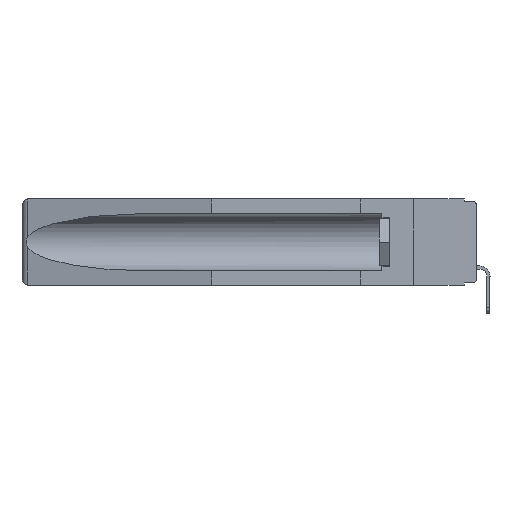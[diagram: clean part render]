
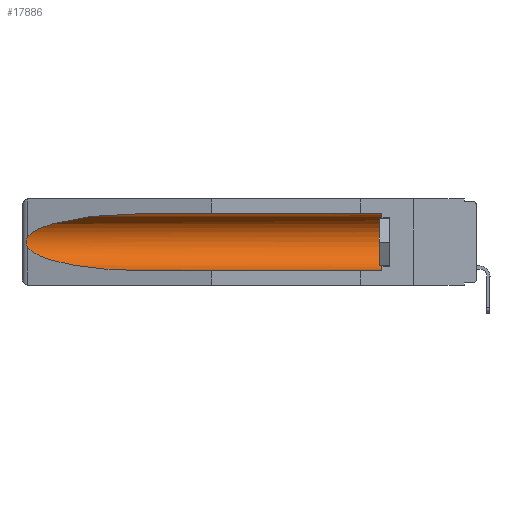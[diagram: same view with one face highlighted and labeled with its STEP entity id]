
A CAD part, left-side view. The second image highlights one B-rep face of the part: STEP entity #17886.
In plain terms, the highlighted cylindrical face has radius 2.857 mm (diameter 5.715 mm), a partial arc.
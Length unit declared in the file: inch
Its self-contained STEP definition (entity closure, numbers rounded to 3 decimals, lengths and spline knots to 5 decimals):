
#38 = AXIS2_PLACEMENT_3D ( 'NONE', #20020, #10484, #16532 ) ;
#1530 = AXIS2_PLACEMENT_3D ( 'NONE', #17863, #13242, #16409 ) ;
#2527 = CARTESIAN_POINT ( 'NONE',  ( 0.26537, 1.52718, -0.19328 ) ) ;
#2916 = ORIENTED_EDGE ( 'NONE', *, *, #14034, .T. ) ;
#3214 = CARTESIAN_POINT ( 'NONE',  ( 0.155, 1.07973, -0.059 ) ) ;
#3494 = LINE ( 'NONE', #19287, #7608 ) ;
#3761 = CARTESIAN_POINT ( 'NONE',  ( 0.21114, 1.30732, -0.284 ) ) ;
#4072 = VERTEX_POINT ( 'NONE', #15041 ) ;
#4190 = EDGE_CURVE ( 'NONE', #12429, #19473, #16996, .T. ) ;
#4382 = DIRECTION ( 'NONE',  ( 0., 1., 0. ) ) ;
#4409 = CARTESIAN_POINT ( 'NONE',  ( 0.2673, 1.53269, -0.17917 ) ) ;
#4736 = CARTESIAN_POINT ( 'NONE',  ( 0.25451, 1.48313, -0.09465 ) ) ;
#4905 = DIRECTION ( 'NONE',  ( 0., 1., 0. ) ) ;
#5392 = VECTOR ( 'NONE', #4382, 39.37008 ) ;
#5512 = CARTESIAN_POINT ( 'NONE',  ( 0.2673, 1.5327, -0.16383 ) ) ;
#5515 = FACE_OUTER_BOUND ( 'NONE', #7435, .T. ) ;
#6349 = ORIENTED_EDGE ( 'NONE', *, *, #6427, .T. ) ;
#6427 = EDGE_CURVE ( 'NONE', #12429, #4072, #8829, .T. ) ;
#6966 = EDGE_CURVE ( 'NONE', #20012, #19473, #16241, .T. ) ;
#7221 = CARTESIAN_POINT ( 'NONE',  ( 0.155, 1.07973, -0.284 ) ) ;
#7435 = EDGE_LOOP ( 'NONE', ( #12212, #15301, #10201, #16638, #6349, #2916 ) ) ;
#7608 = VECTOR ( 'NONE', #4905, 39.37008 ) ;
#7650 = B_SPLINE_CURVE_WITH_KNOTS ( 'NONE', 3,
 ( #10071, #16308, #19599, #5512, #13523, #13426, #4409, #8911, #19697, #14974 ),
 .UNSPECIFIED., .F., .F.,
 ( 4, 2, 2, 2, 4 ),
 ( 0., 0.00029, 0.00058, 0.00087, 0.00117 ),
 .UNSPECIFIED. ) ;
#8364 = CARTESIAN_POINT ( 'NONE',  ( 0.26537, 1.52718, -0.19328 ) ) ;
#8765 = CARTESIAN_POINT ( 'NONE',  ( 0.26537, 1.52718, -0.14972 ) ) ;
#8829 = CIRCLE ( 'NONE', #38, 0.1125 ) ;
#8911 = CARTESIAN_POINT ( 'NONE',  ( 0.26655, 1.53094, -0.18657 ) ) ;
#8990 = CARTESIAN_POINT ( 'NONE',  ( 0.155, -0.30754, -0.284 ) ) ;
#10071 = CARTESIAN_POINT ( 'NONE',  ( 0.26537, 1.52718, -0.14972 ) ) ;
#10201 = ORIENTED_EDGE ( 'NONE', *, *, #6966, .T. ) ;
#10484 = DIRECTION ( 'NONE',  ( 0., -1., 0. ) ) ;
#11089 = EDGE_CURVE ( 'NONE', #14696, #20012, #7650, .T. ) ;
#11600 = CYLINDRICAL_SURFACE ( 'NONE', #1530, 0.1125 ) ;
#12212 = ORIENTED_EDGE ( 'NONE', *, *, #18966, .T. ) ;
#12429 = VERTEX_POINT ( 'NONE', #13427 ) ;
#12685 = VERTEX_POINT ( 'NONE', #12911 ) ;
#12911 = CARTESIAN_POINT ( 'NONE',  ( 0.155, 1.07973, -0.059 ) ) ;
#13242 = DIRECTION ( 'NONE',  ( 0., 1., 0. ) ) ;
#13426 = CARTESIAN_POINT ( 'NONE',  ( 0.2675, 1.53308, -0.17534 ) ) ;
#13427 = CARTESIAN_POINT ( 'NONE',  ( 0.155, 0.126, -0.284 ) ) ;
#13523 = CARTESIAN_POINT ( 'NONE',  ( 0.2675, 1.53308, -0.16763 ) ) ;
#14034 = EDGE_CURVE ( 'NONE', #4072, #12685, #3494, .T. ) ;
#14250 = CARTESIAN_POINT ( 'NONE',  ( 0.155, 1.07973, -0.284 ) ) ;
#14696 = VERTEX_POINT ( 'NONE', #8765 ) ;
#14974 = CARTESIAN_POINT ( 'NONE',  ( 0.26537, 1.52718, -0.19328 ) ) ;
#15041 = CARTESIAN_POINT ( 'NONE',  ( 0.155, 0.126, -0.059 ) ) ;
#15301 = ORIENTED_EDGE ( 'NONE', *, *, #11089, .T. ) ;
#16241 =( BOUNDED_CURVE ( )  B_SPLINE_CURVE ( 3, ( #2527, #16361, #3761, #7221 ),
 .UNSPECIFIED., .F., .F. ) 
 B_SPLINE_CURVE_WITH_KNOTS ( ( 4, 4 ),
 ( 0.1948, 1.5708 ),
 .UNSPECIFIED. ) 
 CURVE ( )  GEOMETRIC_REPRESENTATION_ITEM ( )  RATIONAL_B_SPLINE_CURVE ( ( 1., 0.848, 0.848, 1. ) ) 
 REPRESENTATION_ITEM ( '' )  );
#16308 = CARTESIAN_POINT ( 'NONE',  ( 0.26597, 1.52961, -0.15275 ) ) ;
#16361 = CARTESIAN_POINT ( 'NONE',  ( 0.25451, 1.48313, -0.24835 ) ) ;
#16409 = DIRECTION ( 'NONE',  ( 0., 0., 1. ) ) ;
#16532 = DIRECTION ( 'NONE',  ( 0., 0., 1. ) ) ;
#16638 = ORIENTED_EDGE ( 'NONE', *, *, #4190, .F. ) ;
#16996 = LINE ( 'NONE', #8990, #5392 ) ;
#17255 = CARTESIAN_POINT ( 'NONE',  ( 0.26537, 1.52718, -0.14972 ) ) ;
#17863 = CARTESIAN_POINT ( 'NONE',  ( 0.155, -0.30754, -0.1715 ) ) ;
#17886 = ADVANCED_FACE ( 'NONE', ( #5515 ), #11600, .F. ) ;
#18337 =( BOUNDED_CURVE ( )  B_SPLINE_CURVE ( 3, ( #3214, #18808, #4736, #17255 ),
 .UNSPECIFIED., .F., .F. ) 
 B_SPLINE_CURVE_WITH_KNOTS ( ( 4, 4 ),
 ( 4.71239, 6.08839 ),
 .UNSPECIFIED. ) 
 CURVE ( )  GEOMETRIC_REPRESENTATION_ITEM ( )  RATIONAL_B_SPLINE_CURVE ( ( 1., 0.848, 0.848, 1. ) ) 
 REPRESENTATION_ITEM ( '' )  );
#18808 = CARTESIAN_POINT ( 'NONE',  ( 0.21114, 1.30732, -0.059 ) ) ;
#18966 = EDGE_CURVE ( 'NONE', #12685, #14696, #18337, .T. ) ;
#19287 = CARTESIAN_POINT ( 'NONE',  ( 0.155, -0.30754, -0.059 ) ) ;
#19473 = VERTEX_POINT ( 'NONE', #14250 ) ;
#19599 = CARTESIAN_POINT ( 'NONE',  ( 0.26654, 1.53092, -0.15636 ) ) ;
#19697 = CARTESIAN_POINT ( 'NONE',  ( 0.26597, 1.5296, -0.19026 ) ) ;
#20012 = VERTEX_POINT ( 'NONE', #8364 ) ;
#20020 = CARTESIAN_POINT ( 'NONE',  ( 0.155, 0.126, -0.1715 ) ) ;
